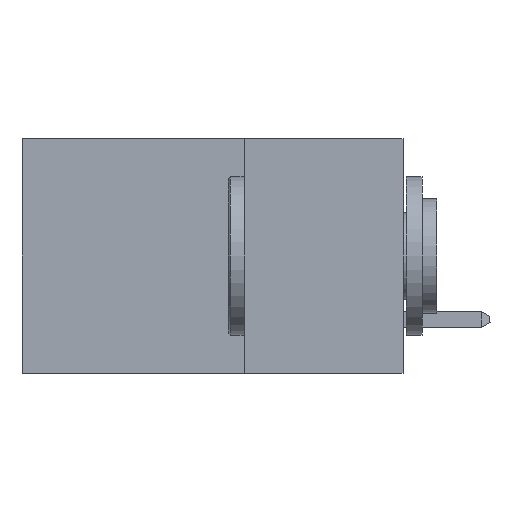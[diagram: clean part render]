
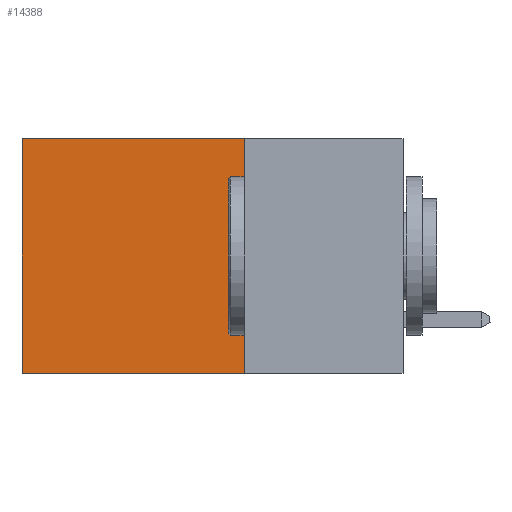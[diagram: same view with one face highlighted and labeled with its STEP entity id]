
A CAD part, left-side view. The second image highlights one B-rep face of the part: STEP entity #14388.
In plain terms, the highlighted planar face has unit normal (-1, 0, 0).
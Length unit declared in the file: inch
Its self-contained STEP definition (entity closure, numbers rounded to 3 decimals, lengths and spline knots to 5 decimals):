
#1061 = LINE ( 'NONE', #20785, #6616 ) ;
#1407 = ORIENTED_EDGE ( 'NONE', *, *, #18443, .T. ) ;
#1690 = VECTOR ( 'NONE', #12552, 39.37008 ) ;
#2480 = EDGE_CURVE ( 'NONE', #12657, #23086, #1061, .T. ) ;
#3174 = DIRECTION ( 'NONE',  ( 0., 1., 0. ) ) ;
#4031 = DIRECTION ( 'NONE',  ( 0., 0., -1. ) ) ;
#4035 = DIRECTION ( 'NONE',  ( 1., 0., 0. ) ) ;
#4905 = EDGE_CURVE ( 'NONE', #9549, #23086, #9907, .T. ) ;
#5522 = CARTESIAN_POINT ( 'NONE',  ( 0.2875, 0.25, 0. ) ) ;
#5786 = CARTESIAN_POINT ( 'NONE',  ( 0.2875, 0.25, -0.37 ) ) ;
#5882 = VECTOR ( 'NONE', #4031, 39.37008 ) ;
#6402 = ORIENTED_EDGE ( 'NONE', *, *, #4905, .T. ) ;
#6616 = VECTOR ( 'NONE', #3174, 39.37008 ) ;
#6683 = EDGE_LOOP ( 'NONE', ( #6402, #11333, #10802, #1407 ) ) ;
#9549 = VERTEX_POINT ( 'NONE', #13435 ) ;
#9907 = LINE ( 'NONE', #11877, #5882 ) ;
#10802 = ORIENTED_EDGE ( 'NONE', *, *, #20354, .F. ) ;
#11333 = ORIENTED_EDGE ( 'NONE', *, *, #2480, .F. ) ;
#11799 = PLANE ( 'NONE',  #17059 ) ;
#11877 = CARTESIAN_POINT ( 'NONE',  ( 0.2875, 0.6, 0. ) ) ;
#12458 = CARTESIAN_POINT ( 'NONE',  ( 0.2875, 0.25, 0. ) ) ;
#12552 = DIRECTION ( 'NONE',  ( 0., 1., 0. ) ) ;
#12657 = VERTEX_POINT ( 'NONE', #5786 ) ;
#13435 = CARTESIAN_POINT ( 'NONE',  ( 0.2875, 0.6, 0. ) ) ;
#13550 = DIRECTION ( 'NONE',  ( 0., 0., -1. ) ) ;
#14388 = ADVANCED_FACE ( 'NONE', ( #22218 ), #11799, .F. ) ;
#16728 = VERTEX_POINT ( 'NONE', #22424 ) ;
#16846 = LINE ( 'NONE', #12458, #1690 ) ;
#17059 = AXIS2_PLACEMENT_3D ( 'NONE', #5522, #4035, #21870 ) ;
#17388 = VECTOR ( 'NONE', #13550, 39.37008 ) ;
#18443 = EDGE_CURVE ( 'NONE', #16728, #9549, #16846, .T. ) ;
#20354 = EDGE_CURVE ( 'NONE', #16728, #12657, #20762, .T. ) ;
#20762 = LINE ( 'NONE', #25289, #17388 ) ;
#20785 = CARTESIAN_POINT ( 'NONE',  ( 0.2875, 0.25, -0.37 ) ) ;
#21870 = DIRECTION ( 'NONE',  ( 0., 0., -1. ) ) ;
#22218 = FACE_OUTER_BOUND ( 'NONE', #6683, .T. ) ;
#22424 = CARTESIAN_POINT ( 'NONE',  ( 0.2875, 0.25, 0. ) ) ;
#23086 = VERTEX_POINT ( 'NONE', #24655 ) ;
#24655 = CARTESIAN_POINT ( 'NONE',  ( 0.2875, 0.6, -0.37 ) ) ;
#25289 = CARTESIAN_POINT ( 'NONE',  ( 0.2875, 0.25, 0. ) ) ;
